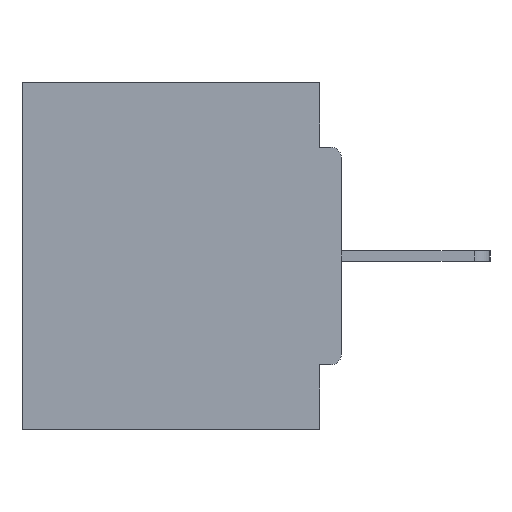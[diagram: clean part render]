
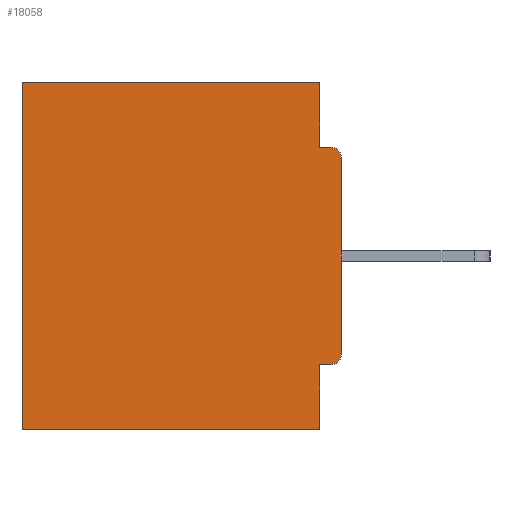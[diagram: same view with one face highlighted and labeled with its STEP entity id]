
A CAD part, left-side view. The second image highlights one B-rep face of the part: STEP entity #18058.
In plain terms, the highlighted planar face has unit normal (-1, 0, 0).
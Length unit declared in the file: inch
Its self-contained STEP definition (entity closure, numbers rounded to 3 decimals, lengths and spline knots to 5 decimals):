
#55 = LINE ( 'NONE', #13536, #6752 ) ;
#174 = AXIS2_PLACEMENT_3D ( 'NONE', #8768, #15216, #22118 ) ;
#302 = CARTESIAN_POINT ( 'NONE',  ( 0.298, 0., -0.1085 ) ) ;
#372 = PLANE ( 'NONE',  #986 ) ;
#912 = ORIENTED_EDGE ( 'NONE', *, *, #11758, .T. ) ;
#986 = AXIS2_PLACEMENT_3D ( 'NONE', #17868, #4545, #11257 ) ;
#1288 = VECTOR ( 'NONE', #17321, 39.37008 ) ;
#1607 = DIRECTION ( 'NONE',  ( 0., 1., 0. ) ) ;
#2408 = VECTOR ( 'NONE', #1607, 39.37008 ) ;
#2576 = DIRECTION ( 'NONE',  ( 0., 0., -1. ) ) ;
#2671 = VERTEX_POINT ( 'NONE', #20190 ) ;
#2803 = DIRECTION ( 'NONE',  ( 0., 1., 0. ) ) ;
#3863 = CIRCLE ( 'NONE', #174, 0.015 ) ;
#4185 = CARTESIAN_POINT ( 'NONE',  ( 0.298, 0.46, 0. ) ) ;
#4545 = DIRECTION ( 'NONE',  ( 1., 0., 0. ) ) ;
#4651 = EDGE_CURVE ( 'NONE', #12977, #9853, #11764, .T. ) ;
#4792 = CARTESIAN_POINT ( 'NONE',  ( 0.298, 0., -0.4065 ) ) ;
#4876 = LINE ( 'NONE', #22961, #9526 ) ;
#4938 = DIRECTION ( 'NONE',  ( 0., 1., 0. ) ) ;
#5012 = ORIENTED_EDGE ( 'NONE', *, *, #11431, .F. ) ;
#5513 = VECTOR ( 'NONE', #26716, 39.37008 ) ;
#5652 = CARTESIAN_POINT ( 'NONE',  ( 0.298, 0.031, -0.4065 ) ) ;
#6752 = VECTOR ( 'NONE', #4938, 39.37008 ) ;
#7195 = CARTESIAN_POINT ( 'NONE',  ( 0.298, 0., -0.0935 ) ) ;
#7593 = EDGE_LOOP ( 'NONE', ( #27793, #16087, #22893, #912, #28324, #19932, #21441, #14557, #22466, #5012 ) ) ;
#8330 = CARTESIAN_POINT ( 'NONE',  ( 0.298, 0., -0.5 ) ) ;
#8466 = EDGE_CURVE ( 'NONE', #20604, #2671, #25250, .T. ) ;
#8740 = EDGE_CURVE ( 'NONE', #18790, #9853, #10818, .T. ) ;
#8768 = CARTESIAN_POINT ( 'NONE',  ( 0.298, 0.015, -0.3915 ) ) ;
#9094 = LINE ( 'NONE', #4792, #13599 ) ;
#9319 = CARTESIAN_POINT ( 'NONE',  ( 0.298, 0.46, 0. ) ) ;
#9405 = VERTEX_POINT ( 'NONE', #5652 ) ;
#9526 = VECTOR ( 'NONE', #13621, 39.37008 ) ;
#9853 = VERTEX_POINT ( 'NONE', #12366 ) ;
#9864 = VERTEX_POINT ( 'NONE', #25162 ) ;
#9880 = DIRECTION ( 'NONE',  ( 0., 0., -1. ) ) ;
#10818 = CIRCLE ( 'NONE', #15870, 0.015 ) ;
#11257 = DIRECTION ( 'NONE',  ( 0., 0., -1. ) ) ;
#11431 = EDGE_CURVE ( 'NONE', #18790, #20212, #13153, .T. ) ;
#11758 = EDGE_CURVE ( 'NONE', #11848, #20604, #55, .T. ) ;
#11764 = LINE ( 'NONE', #7195, #5513 ) ;
#11794 = EDGE_CURVE ( 'NONE', #9864, #9405, #9094, .T. ) ;
#11848 = VERTEX_POINT ( 'NONE', #22313 ) ;
#11973 = EDGE_CURVE ( 'NONE', #9405, #23642, #20854, .T. ) ;
#12366 = CARTESIAN_POINT ( 'NONE',  ( 0.298, 0.015, -0.0935 ) ) ;
#12773 = EDGE_CURVE ( 'NONE', #11848, #12977, #4876, .T. ) ;
#12977 = VERTEX_POINT ( 'NONE', #18647 ) ;
#13153 = LINE ( 'NONE', #15447, #1288 ) ;
#13536 = CARTESIAN_POINT ( 'NONE',  ( 0.298, 0., 0. ) ) ;
#13599 = VECTOR ( 'NONE', #2803, 39.37008 ) ;
#13621 = DIRECTION ( 'NONE',  ( 0., 0., -1. ) ) ;
#14555 = CARTESIAN_POINT ( 'NONE',  ( 0.298, 0., -0.3915 ) ) ;
#14557 = ORIENTED_EDGE ( 'NONE', *, *, #11794, .F. ) ;
#15216 = DIRECTION ( 'NONE',  ( -1., 0., 0. ) ) ;
#15447 = CARTESIAN_POINT ( 'NONE',  ( 0.298, 0., 0. ) ) ;
#15870 = AXIS2_PLACEMENT_3D ( 'NONE', #23950, #19484, #2576 ) ;
#16087 = ORIENTED_EDGE ( 'NONE', *, *, #4651, .F. ) ;
#16253 = DIRECTION ( 'NONE',  ( 0., 0., -1. ) ) ;
#17309 = FACE_OUTER_BOUND ( 'NONE', #7593, .T. ) ;
#17321 = DIRECTION ( 'NONE',  ( 0., 0., -1. ) ) ;
#17868 = CARTESIAN_POINT ( 'NONE',  ( 0.298, 0., 0. ) ) ;
#18058 = ADVANCED_FACE ( 'NONE', ( #17309 ), #372, .F. ) ;
#18647 = CARTESIAN_POINT ( 'NONE',  ( 0.298, 0.031, -0.0935 ) ) ;
#18709 = CARTESIAN_POINT ( 'NONE',  ( 0.298, 0.031, -0.5 ) ) ;
#18790 = VERTEX_POINT ( 'NONE', #302 ) ;
#19484 = DIRECTION ( 'NONE',  ( -1., 0., 0. ) ) ;
#19932 = ORIENTED_EDGE ( 'NONE', *, *, #25233, .F. ) ;
#19983 = VECTOR ( 'NONE', #9880, 39.37008 ) ;
#20190 = CARTESIAN_POINT ( 'NONE',  ( 0.298, 0.46, -0.5 ) ) ;
#20212 = VERTEX_POINT ( 'NONE', #14555 ) ;
#20604 = VERTEX_POINT ( 'NONE', #4185 ) ;
#20854 = LINE ( 'NONE', #18709, #26472 ) ;
#21399 = LINE ( 'NONE', #8330, #2408 ) ;
#21441 = ORIENTED_EDGE ( 'NONE', *, *, #11973, .F. ) ;
#22100 = EDGE_CURVE ( 'NONE', #9864, #20212, #3863, .T. ) ;
#22118 = DIRECTION ( 'NONE',  ( 0., 0., -1. ) ) ;
#22313 = CARTESIAN_POINT ( 'NONE',  ( 0.298, 0.031, 0. ) ) ;
#22377 = CARTESIAN_POINT ( 'NONE',  ( 0.298, 0.031, -0.5 ) ) ;
#22466 = ORIENTED_EDGE ( 'NONE', *, *, #22100, .T. ) ;
#22893 = ORIENTED_EDGE ( 'NONE', *, *, #12773, .F. ) ;
#22961 = CARTESIAN_POINT ( 'NONE',  ( 0.298, 0.031, -0.5 ) ) ;
#23642 = VERTEX_POINT ( 'NONE', #22377 ) ;
#23950 = CARTESIAN_POINT ( 'NONE',  ( 0.298, 0.015, -0.1085 ) ) ;
#25162 = CARTESIAN_POINT ( 'NONE',  ( 0.298, 0.015, -0.4065 ) ) ;
#25233 = EDGE_CURVE ( 'NONE', #23642, #2671, #21399, .T. ) ;
#25250 = LINE ( 'NONE', #9319, #19983 ) ;
#26472 = VECTOR ( 'NONE', #16253, 39.37008 ) ;
#26716 = DIRECTION ( 'NONE',  ( 0., -1., 0. ) ) ;
#27793 = ORIENTED_EDGE ( 'NONE', *, *, #8740, .T. ) ;
#28324 = ORIENTED_EDGE ( 'NONE', *, *, #8466, .T. ) ;
